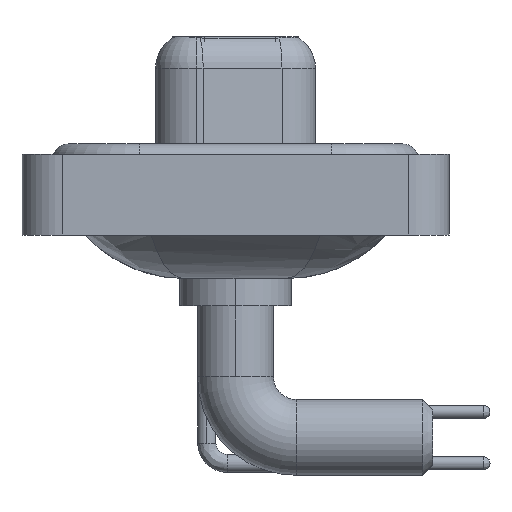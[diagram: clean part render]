
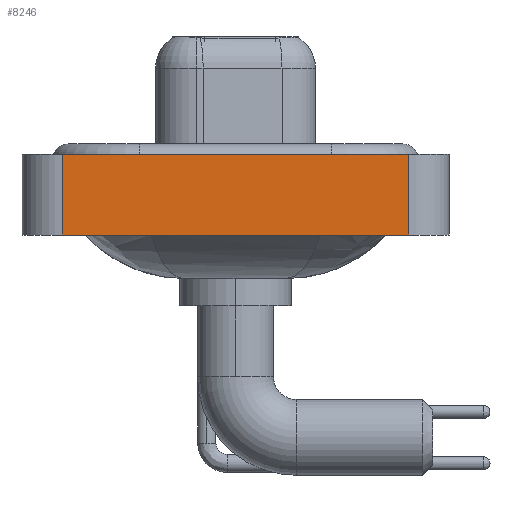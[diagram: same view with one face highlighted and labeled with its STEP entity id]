
A CAD part, left-side view. The second image highlights one B-rep face of the part: STEP entity #8246.
In plain terms, the highlighted planar face has unit normal (-1, 0, 0).
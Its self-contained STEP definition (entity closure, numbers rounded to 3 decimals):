
#37 = DIRECTION ( 'NONE',  ( 0., 0., 1. ) ) ;
#1763 = VECTOR ( 'NONE', #10946, 1000. ) ;
#3315 = FACE_OUTER_BOUND ( 'NONE', #21993, .T. ) ;
#3352 = CARTESIAN_POINT ( 'NONE',  ( -7.35, -8.55, 0.4 ) ) ;
#4182 = EDGE_CURVE ( 'NONE', #17516, #7663, #15311, .T. ) ;
#4806 = ORIENTED_EDGE ( 'NONE', *, *, #7039, .F. ) ;
#5271 = CARTESIAN_POINT ( 'NONE',  ( -7.35, -8.55, -3.6 ) ) ;
#6829 = EDGE_CURVE ( 'NONE', #22724, #17516, #13560, .T. ) ;
#7039 = EDGE_CURVE ( 'NONE', #22724, #9050, #9506, .T. ) ;
#7663 = VERTEX_POINT ( 'NONE', #23245 ) ;
#8246 = ADVANCED_FACE ( 'NONE', ( #3315 ), #9017, .T. ) ;
#8938 = ORIENTED_EDGE ( 'NONE', *, *, #24274, .F. ) ;
#9017 = PLANE ( 'NONE',  #11822 ) ;
#9050 = VERTEX_POINT ( 'NONE', #24238 ) ;
#9364 = ORIENTED_EDGE ( 'NONE', *, *, #6829, .T. ) ;
#9506 = LINE ( 'NONE', #16699, #16139 ) ;
#9688 = DIRECTION ( 'NONE',  ( 0., -1., 0. ) ) ;
#10051 = VECTOR ( 'NONE', #24525, 1000. ) ;
#10555 = VECTOR ( 'NONE', #9688, 1000. ) ;
#10946 = DIRECTION ( 'NONE',  ( 0., -1., 0. ) ) ;
#11822 = AXIS2_PLACEMENT_3D ( 'NONE', #5271, #16461, #18462 ) ;
#13560 = LINE ( 'NONE', #21228, #10555 ) ;
#15311 = LINE ( 'NONE', #16928, #10051 ) ;
#16104 = CARTESIAN_POINT ( 'NONE',  ( -7.35, -8.55, -3.6 ) ) ;
#16139 = VECTOR ( 'NONE', #37, 1000. ) ;
#16271 = ORIENTED_EDGE ( 'NONE', *, *, #4182, .T. ) ;
#16461 = DIRECTION ( 'NONE',  ( -1., 0., 0. ) ) ;
#16699 = CARTESIAN_POINT ( 'NONE',  ( -7.35, 8.55, -3.6 ) ) ;
#16928 = CARTESIAN_POINT ( 'NONE',  ( -7.35, -8.55, -3.6 ) ) ;
#17516 = VERTEX_POINT ( 'NONE', #16104 ) ;
#18462 = DIRECTION ( 'NONE',  ( 0., 0., 1. ) ) ;
#21228 = CARTESIAN_POINT ( 'NONE',  ( -7.35, -8.55, -3.6 ) ) ;
#21993 = EDGE_LOOP ( 'NONE', ( #16271, #8938, #4806, #9364 ) ) ;
#22106 = CARTESIAN_POINT ( 'NONE',  ( -7.35, 8.55, -3.6 ) ) ;
#22724 = VERTEX_POINT ( 'NONE', #22106 ) ;
#23245 = CARTESIAN_POINT ( 'NONE',  ( -7.35, -8.55, 0.4 ) ) ;
#24238 = CARTESIAN_POINT ( 'NONE',  ( -7.35, 8.55, 0.4 ) ) ;
#24274 = EDGE_CURVE ( 'NONE', #9050, #7663, #24457, .T. ) ;
#24457 = LINE ( 'NONE', #3352, #1763 ) ;
#24525 = DIRECTION ( 'NONE',  ( 0., 0., 1. ) ) ;
